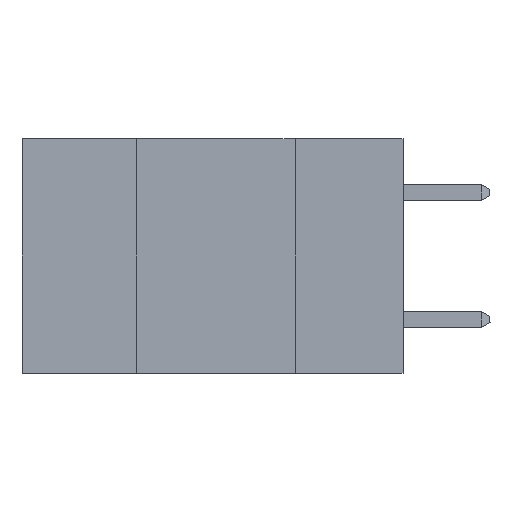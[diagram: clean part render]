
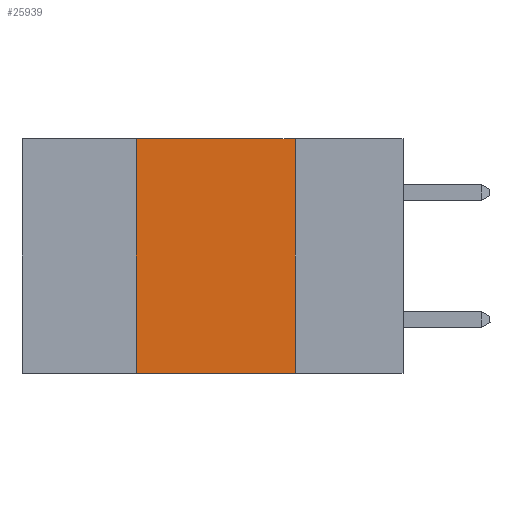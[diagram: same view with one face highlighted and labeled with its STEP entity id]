
A CAD part, left-side view. The second image highlights one B-rep face of the part: STEP entity #25939.
In plain terms, the highlighted planar face has unit normal (-1, 0, 0).
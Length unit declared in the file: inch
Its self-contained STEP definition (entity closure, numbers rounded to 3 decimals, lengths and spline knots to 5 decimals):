
#478 = CARTESIAN_POINT ( 'NONE',  ( 0., 0.17, -0.37 ) ) ;
#758 = ORIENTED_EDGE ( 'NONE', *, *, #20701, .F. ) ;
#2435 = PLANE ( 'NONE',  #2645 ) ;
#2645 = AXIS2_PLACEMENT_3D ( 'NONE', #14140, #16829, #13838 ) ;
#3127 = CARTESIAN_POINT ( 'NONE',  ( 0., 0.6, -0.37 ) ) ;
#3144 = CARTESIAN_POINT ( 'NONE',  ( 0., 0.42, -0.37 ) ) ;
#3233 = LINE ( 'NONE', #14046, #9895 ) ;
#4020 = CARTESIAN_POINT ( 'NONE',  ( 0., 0.6, 0. ) ) ;
#5841 = EDGE_CURVE ( 'NONE', #16973, #19948, #14240, .T. ) ;
#6143 = ORIENTED_EDGE ( 'NONE', *, *, #21486, .F. ) ;
#7233 = CARTESIAN_POINT ( 'NONE',  ( 0., 0.42, 0. ) ) ;
#7859 = CARTESIAN_POINT ( 'NONE',  ( 0., 0.42, 0. ) ) ;
#8328 = VECTOR ( 'NONE', #23385, 39.37008 ) ;
#8618 = EDGE_CURVE ( 'NONE', #17431, #19948, #3233, .T. ) ;
#9895 = VECTOR ( 'NONE', #11948, 39.37008 ) ;
#10081 = EDGE_LOOP ( 'NONE', ( #19957, #758, #6143, #28224 ) ) ;
#10717 = VERTEX_POINT ( 'NONE', #7233 ) ;
#11948 = DIRECTION ( 'NONE',  ( 0., 0., -1. ) ) ;
#13838 = DIRECTION ( 'NONE',  ( 0., 0., -1. ) ) ;
#14046 = CARTESIAN_POINT ( 'NONE',  ( 0., 0.17, 0. ) ) ;
#14140 = CARTESIAN_POINT ( 'NONE',  ( 0., 0.6, 0. ) ) ;
#14240 = LINE ( 'NONE', #3127, #8328 ) ;
#16829 = DIRECTION ( 'NONE',  ( 1., 0., 0. ) ) ;
#16973 = VERTEX_POINT ( 'NONE', #3144 ) ;
#17001 = DIRECTION ( 'NONE',  ( 0., 0., 1. ) ) ;
#17431 = VERTEX_POINT ( 'NONE', #29083 ) ;
#18104 = DIRECTION ( 'NONE',  ( 0., -1., 0. ) ) ;
#19948 = VERTEX_POINT ( 'NONE', #478 ) ;
#19957 = ORIENTED_EDGE ( 'NONE', *, *, #8618, .F. ) ;
#20701 = EDGE_CURVE ( 'NONE', #10717, #17431, #24579, .T. ) ;
#21486 = EDGE_CURVE ( 'NONE', #16973, #10717, #28432, .T. ) ;
#23385 = DIRECTION ( 'NONE',  ( 0., -1., 0. ) ) ;
#24562 = VECTOR ( 'NONE', #18104, 39.37008 ) ;
#24579 = LINE ( 'NONE', #4020, #24562 ) ;
#25939 = ADVANCED_FACE ( 'NONE', ( #27953 ), #2435, .F. ) ;
#27953 = FACE_OUTER_BOUND ( 'NONE', #10081, .T. ) ;
#28224 = ORIENTED_EDGE ( 'NONE', *, *, #5841, .T. ) ;
#28432 = LINE ( 'NONE', #7859, #29412 ) ;
#29083 = CARTESIAN_POINT ( 'NONE',  ( 0., 0.17, 0. ) ) ;
#29412 = VECTOR ( 'NONE', #17001, 39.37008 ) ;
